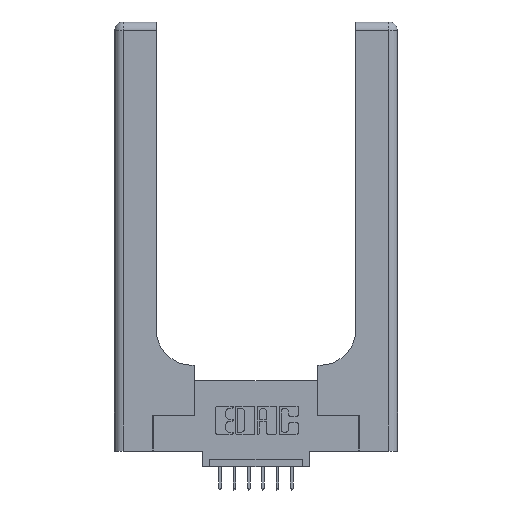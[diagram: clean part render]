
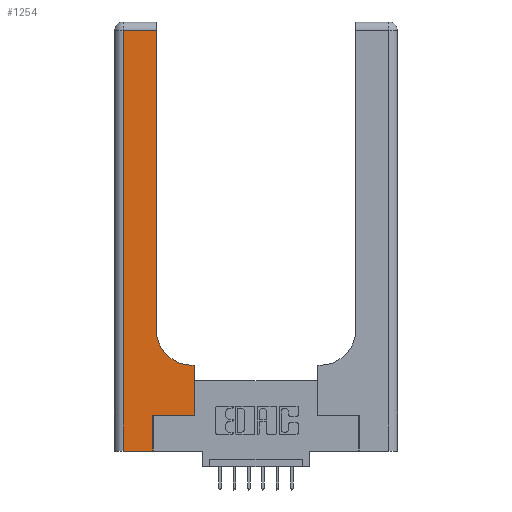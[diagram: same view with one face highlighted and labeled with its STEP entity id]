
A CAD part, top view. The second image highlights one B-rep face of the part: STEP entity #1254.
In plain terms, the highlighted planar face has unit normal (0, 0, 1).
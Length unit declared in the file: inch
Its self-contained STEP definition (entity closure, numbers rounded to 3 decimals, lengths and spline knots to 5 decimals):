
#79 = ORIENTED_EDGE ( 'NONE', *, *, #8078, .T. ) ;
#232 = DIRECTION ( 'NONE',  ( 1., 0., 0. ) ) ;
#310 = DIRECTION ( 'NONE',  ( 1., 0., 0. ) ) ;
#430 = DIRECTION ( 'NONE',  ( 0., 1., 0. ) ) ;
#605 = LINE ( 'NONE', #6273, #7587 ) ;
#726 = LINE ( 'NONE', #11709, #9679 ) ;
#768 = ORIENTED_EDGE ( 'NONE', *, *, #8518, .T. ) ;
#916 = CARTESIAN_POINT ( 'NONE',  ( 0.5415, 0.85, 0.37 ) ) ;
#1098 = CARTESIAN_POINT ( 'NONE',  ( 0.269, 0.25, 0.37 ) ) ;
#1254 = ADVANCED_FACE ( 'NONE', ( #13824 ), #13871, .F. ) ;
#1267 = VERTEX_POINT ( 'NONE', #2481 ) ;
#1772 = LINE ( 'NONE', #2442, #10743 ) ;
#1966 = DIRECTION ( 'NONE',  ( -1., 0., 0. ) ) ;
#2072 = EDGE_CURVE ( 'NONE', #1267, #11682, #605, .T. ) ;
#2442 = CARTESIAN_POINT ( 'NONE',  ( 0., 0., 0.37 ) ) ;
#2481 = CARTESIAN_POINT ( 'NONE',  ( 0.2915, 0.85, 0.37 ) ) ;
#2703 = VERTEX_POINT ( 'NONE', #13005 ) ;
#3097 = DIRECTION ( 'NONE',  ( 0., 0., -1. ) ) ;
#3136 = CARTESIAN_POINT ( 'NONE',  ( 0.5585, 0.6, 0.37 ) ) ;
#3137 = CARTESIAN_POINT ( 'NONE',  ( 0.269, 0., 0.37 ) ) ;
#3662 = ORIENTED_EDGE ( 'NONE', *, *, #8251, .T. ) ;
#3974 = ORIENTED_EDGE ( 'NONE', *, *, #11573, .T. ) ;
#4087 = VECTOR ( 'NONE', #5573, 39.37008 ) ;
#4211 = VECTOR ( 'NONE', #12604, 39.37008 ) ;
#4243 = VERTEX_POINT ( 'NONE', #1098 ) ;
#4274 = DIRECTION ( 'NONE',  ( 0., 1., 0. ) ) ;
#4597 = CARTESIAN_POINT ( 'NONE',  ( 0.2915, 0.6, 0.37 ) ) ;
#4644 = LINE ( 'NONE', #3137, #14616 ) ;
#4683 = AXIS2_PLACEMENT_3D ( 'NONE', #9284, #4805, #9435 ) ;
#4805 = DIRECTION ( 'NONE',  ( 0., 0., -1. ) ) ;
#4929 = VERTEX_POINT ( 'NONE', #3136 ) ;
#4980 = ORIENTED_EDGE ( 'NONE', *, *, #5476, .T. ) ;
#5476 = EDGE_CURVE ( 'NONE', #5650, #4243, #4644, .T. ) ;
#5501 = VECTOR ( 'NONE', #310, 39.37008 ) ;
#5573 = DIRECTION ( 'NONE',  ( 0., -1., 0. ) ) ;
#5650 = VERTEX_POINT ( 'NONE', #7843 ) ;
#6273 = CARTESIAN_POINT ( 'NONE',  ( 0.2915, 3., 0.37 ) ) ;
#7133 = VECTOR ( 'NONE', #1966, 39.37008 ) ;
#7179 = CARTESIAN_POINT ( 'NONE',  ( 0.269, 0.25, 0.37 ) ) ;
#7587 = VECTOR ( 'NONE', #430, 39.37008 ) ;
#7843 = CARTESIAN_POINT ( 'NONE',  ( 0.269, 0., 0.37 ) ) ;
#8078 = EDGE_CURVE ( 'NONE', #11471, #1267, #11036, .T. ) ;
#8251 = EDGE_CURVE ( 'NONE', #4243, #2703, #11563, .T. ) ;
#8518 = EDGE_CURVE ( 'NONE', #11682, #11249, #14371, .T. ) ;
#8538 = LINE ( 'NONE', #4597, #4211 ) ;
#8849 = CARTESIAN_POINT ( 'NONE',  ( 0., 2.94, 0.37 ) ) ;
#9284 = CARTESIAN_POINT ( 'NONE',  ( 0., 3., 0.37 ) ) ;
#9389 = AXIS2_PLACEMENT_3D ( 'NONE', #916, #3097, #12248 ) ;
#9435 = DIRECTION ( 'NONE',  ( -1., 0., 0. ) ) ;
#9441 = CARTESIAN_POINT ( 'NONE',  ( 0.2915, 2.94, 0.37 ) ) ;
#9679 = VECTOR ( 'NONE', #12862, 39.37008 ) ;
#10371 = ORIENTED_EDGE ( 'NONE', *, *, #14370, .T. ) ;
#10743 = VECTOR ( 'NONE', #232, 39.37008 ) ;
#11036 = CIRCLE ( 'NONE', #9389, 0.25 ) ;
#11063 = LINE ( 'NONE', #12470, #4087 ) ;
#11249 = VERTEX_POINT ( 'NONE', #11756 ) ;
#11270 = EDGE_CURVE ( 'NONE', #2703, #4929, #726, .T. ) ;
#11471 = VERTEX_POINT ( 'NONE', #12080 ) ;
#11510 = VERTEX_POINT ( 'NONE', #13541 ) ;
#11563 = LINE ( 'NONE', #7179, #5501 ) ;
#11573 = EDGE_CURVE ( 'NONE', #11510, #5650, #1772, .T. ) ;
#11646 = ORIENTED_EDGE ( 'NONE', *, *, #11270, .T. ) ;
#11682 = VERTEX_POINT ( 'NONE', #9441 ) ;
#11709 = CARTESIAN_POINT ( 'NONE',  ( 0.5585, 0.25, 0.37 ) ) ;
#11756 = CARTESIAN_POINT ( 'NONE',  ( 0.06, 2.94, 0.37 ) ) ;
#12080 = CARTESIAN_POINT ( 'NONE',  ( 0.5415, 0.6, 0.37 ) ) ;
#12131 = EDGE_CURVE ( 'NONE', #11249, #11510, #11063, .T. ) ;
#12248 = DIRECTION ( 'NONE',  ( 1., 0., 0. ) ) ;
#12470 = CARTESIAN_POINT ( 'NONE',  ( 0.06, 3., 0.37 ) ) ;
#12604 = DIRECTION ( 'NONE',  ( -1., 0., 0. ) ) ;
#12850 = EDGE_LOOP ( 'NONE', ( #14064, #768, #14318, #3974, #4980, #3662, #11646, #10371, #79 ) ) ;
#12862 = DIRECTION ( 'NONE',  ( 0., 1., 0. ) ) ;
#13005 = CARTESIAN_POINT ( 'NONE',  ( 0.5585, 0.25, 0.37 ) ) ;
#13541 = CARTESIAN_POINT ( 'NONE',  ( 0.06, 0., 0.37 ) ) ;
#13824 = FACE_OUTER_BOUND ( 'NONE', #12850, .T. ) ;
#13871 = PLANE ( 'NONE',  #4683 ) ;
#14064 = ORIENTED_EDGE ( 'NONE', *, *, #2072, .T. ) ;
#14318 = ORIENTED_EDGE ( 'NONE', *, *, #12131, .T. ) ;
#14370 = EDGE_CURVE ( 'NONE', #4929, #11471, #8538, .T. ) ;
#14371 = LINE ( 'NONE', #8849, #7133 ) ;
#14616 = VECTOR ( 'NONE', #4274, 39.37008 ) ;
